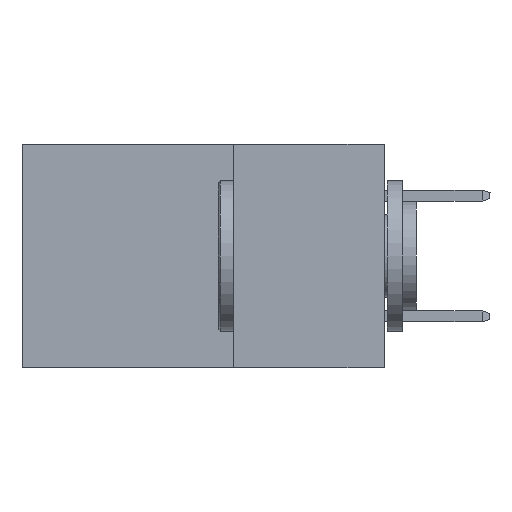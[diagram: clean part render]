
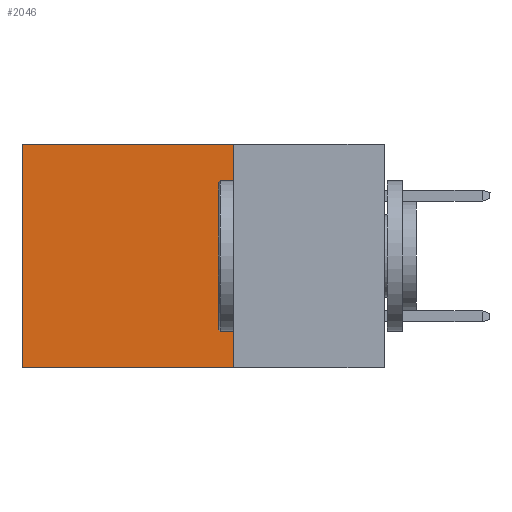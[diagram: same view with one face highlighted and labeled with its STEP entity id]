
A CAD part, left-side view. The second image highlights one B-rep face of the part: STEP entity #2046.
In plain terms, the highlighted planar face has unit normal (-1, 0, 0).
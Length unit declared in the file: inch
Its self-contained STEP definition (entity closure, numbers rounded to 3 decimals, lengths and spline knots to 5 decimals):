
#131 = CARTESIAN_POINT ( 'NONE',  ( 0.298, 0.6, 0. ) ) ;
#2046 = ADVANCED_FACE ( 'NONE', ( #4947 ), #21118, .F. ) ;
#2177 = ORIENTED_EDGE ( 'NONE', *, *, #5611, .T. ) ;
#3233 = DIRECTION ( 'NONE',  ( 0., 0., -1. ) ) ;
#3719 = VERTEX_POINT ( 'NONE', #22351 ) ;
#3909 = CARTESIAN_POINT ( 'NONE',  ( 0.298, 0.25, -0.37 ) ) ;
#4678 = CARTESIAN_POINT ( 'NONE',  ( 0.298, 0.25, -0.37 ) ) ;
#4947 = FACE_OUTER_BOUND ( 'NONE', #7736, .T. ) ;
#5611 = EDGE_CURVE ( 'NONE', #10335, #11152, #13526, .T. ) ;
#5802 = CARTESIAN_POINT ( 'NONE',  ( 0.298, 0.25, 0. ) ) ;
#6877 = DIRECTION ( 'NONE',  ( 1., 0., 0. ) ) ;
#7059 = ORIENTED_EDGE ( 'NONE', *, *, #12592, .F. ) ;
#7498 = AXIS2_PLACEMENT_3D ( 'NONE', #11236, #6877, #25391 ) ;
#7736 = EDGE_LOOP ( 'NONE', ( #8585, #7059, #12506, #2177 ) ) ;
#8585 = ORIENTED_EDGE ( 'NONE', *, *, #24549, .T. ) ;
#8857 = LINE ( 'NONE', #131, #9182 ) ;
#9182 = VECTOR ( 'NONE', #12303, 39.37008 ) ;
#10136 = LINE ( 'NONE', #15369, #22146 ) ;
#10335 = VERTEX_POINT ( 'NONE', #12814 ) ;
#11152 = VERTEX_POINT ( 'NONE', #11317 ) ;
#11236 = CARTESIAN_POINT ( 'NONE',  ( 0.298, 0.25, 0. ) ) ;
#11317 = CARTESIAN_POINT ( 'NONE',  ( 0.298, 0.6, 0. ) ) ;
#11992 = DIRECTION ( 'NONE',  ( 0., 1., 0. ) ) ;
#12303 = DIRECTION ( 'NONE',  ( 0., 0., -1. ) ) ;
#12506 = ORIENTED_EDGE ( 'NONE', *, *, #13036, .F. ) ;
#12592 = EDGE_CURVE ( 'NONE', #14630, #3719, #19661, .T. ) ;
#12814 = CARTESIAN_POINT ( 'NONE',  ( 0.298, 0.25, 0. ) ) ;
#13036 = EDGE_CURVE ( 'NONE', #10335, #14630, #10136, .T. ) ;
#13526 = LINE ( 'NONE', #5802, #14784 ) ;
#14630 = VERTEX_POINT ( 'NONE', #3909 ) ;
#14688 = DIRECTION ( 'NONE',  ( 0., 1., 0. ) ) ;
#14784 = VECTOR ( 'NONE', #11992, 39.37008 ) ;
#15369 = CARTESIAN_POINT ( 'NONE',  ( 0.298, 0.25, 0. ) ) ;
#17148 = VECTOR ( 'NONE', #14688, 39.37008 ) ;
#19661 = LINE ( 'NONE', #4678, #17148 ) ;
#21118 = PLANE ( 'NONE',  #7498 ) ;
#22146 = VECTOR ( 'NONE', #3233, 39.37008 ) ;
#22351 = CARTESIAN_POINT ( 'NONE',  ( 0.298, 0.6, -0.37 ) ) ;
#24549 = EDGE_CURVE ( 'NONE', #11152, #3719, #8857, .T. ) ;
#25391 = DIRECTION ( 'NONE',  ( 0., 0., -1. ) ) ;
